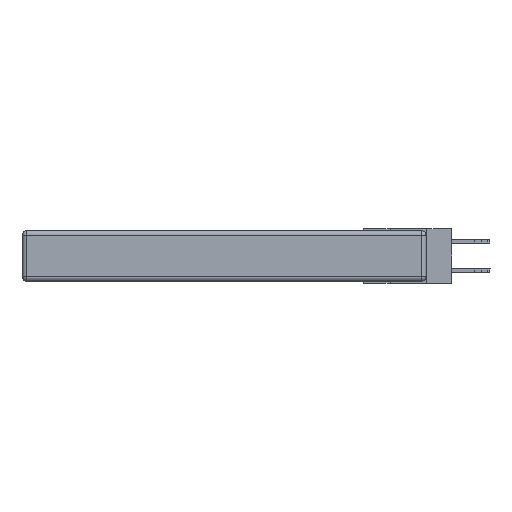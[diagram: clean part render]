
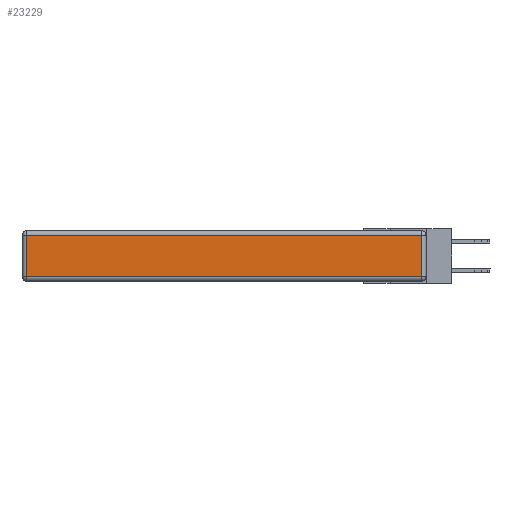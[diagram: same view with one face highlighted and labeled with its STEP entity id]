
A CAD part, left-side view. The second image highlights one B-rep face of the part: STEP entity #23229.
In plain terms, the highlighted planar face has unit normal (-1, 0, 0).
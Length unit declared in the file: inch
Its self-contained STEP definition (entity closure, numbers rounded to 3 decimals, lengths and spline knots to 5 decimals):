
#1112 = CARTESIAN_POINT ( 'NONE',  ( 0., 0.03, -0.03 ) ) ;
#1231 = AXIS2_PLACEMENT_3D ( 'NONE', #11388, #26807, #24443 ) ;
#1836 = VECTOR ( 'NONE', #15608, 39.37008 ) ;
#1843 = EDGE_CURVE ( 'NONE', #10730, #16482, #5734, .T. ) ;
#2300 = ORIENTED_EDGE ( 'NONE', *, *, #3954, .T. ) ;
#2674 = VERTEX_POINT ( 'NONE', #5470 ) ;
#2802 = ORIENTED_EDGE ( 'NONE', *, *, #1843, .T. ) ;
#3954 = EDGE_CURVE ( 'NONE', #16482, #25564, #12524, .T. ) ;
#5470 = CARTESIAN_POINT ( 'NONE',  ( 0., 2.72, -0.03 ) ) ;
#5734 = LINE ( 'NONE', #15690, #1836 ) ;
#6105 = CARTESIAN_POINT ( 'NONE',  ( 0., 0.03, -0.343 ) ) ;
#7801 = LINE ( 'NONE', #10573, #14004 ) ;
#8754 = CARTESIAN_POINT ( 'NONE',  ( 0., 0.03, -0.313 ) ) ;
#9261 = CARTESIAN_POINT ( 'NONE',  ( 0., 2.72, -0.313 ) ) ;
#10573 = CARTESIAN_POINT ( 'NONE',  ( 0., 2.72, -0.343 ) ) ;
#10730 = VERTEX_POINT ( 'NONE', #9261 ) ;
#10746 = PLANE ( 'NONE',  #1231 ) ;
#11388 = CARTESIAN_POINT ( 'NONE',  ( 0., 0., -0.343 ) ) ;
#12524 = LINE ( 'NONE', #6105, #25259 ) ;
#12590 = DIRECTION ( 'NONE',  ( 0., 0., 1. ) ) ;
#12832 = DIRECTION ( 'NONE',  ( 0., 0., -1. ) ) ;
#14004 = VECTOR ( 'NONE', #12832, 39.37008 ) ;
#15608 = DIRECTION ( 'NONE',  ( 0., -1., 0. ) ) ;
#15690 = CARTESIAN_POINT ( 'NONE',  ( 0., 0., -0.313 ) ) ;
#16482 = VERTEX_POINT ( 'NONE', #8754 ) ;
#17041 = EDGE_CURVE ( 'NONE', #2674, #10730, #7801, .T. ) ;
#17176 = FACE_OUTER_BOUND ( 'NONE', #24580, .T. ) ;
#19328 = EDGE_CURVE ( 'NONE', #25564, #2674, #26397, .T. ) ;
#20866 = VECTOR ( 'NONE', #25333, 39.37008 ) ;
#21047 = CARTESIAN_POINT ( 'NONE',  ( 0., 2.75, -0.03 ) ) ;
#21810 = ORIENTED_EDGE ( 'NONE', *, *, #17041, .T. ) ;
#23229 = ADVANCED_FACE ( 'NONE', ( #17176 ), #10746, .T. ) ;
#23933 = ORIENTED_EDGE ( 'NONE', *, *, #19328, .T. ) ;
#24443 = DIRECTION ( 'NONE',  ( 0., 0., 1. ) ) ;
#24580 = EDGE_LOOP ( 'NONE', ( #2802, #2300, #23933, #21810 ) ) ;
#25259 = VECTOR ( 'NONE', #12590, 39.37008 ) ;
#25333 = DIRECTION ( 'NONE',  ( 0., 1., 0. ) ) ;
#25564 = VERTEX_POINT ( 'NONE', #1112 ) ;
#26397 = LINE ( 'NONE', #21047, #20866 ) ;
#26807 = DIRECTION ( 'NONE',  ( -1., 0., 0. ) ) ;
